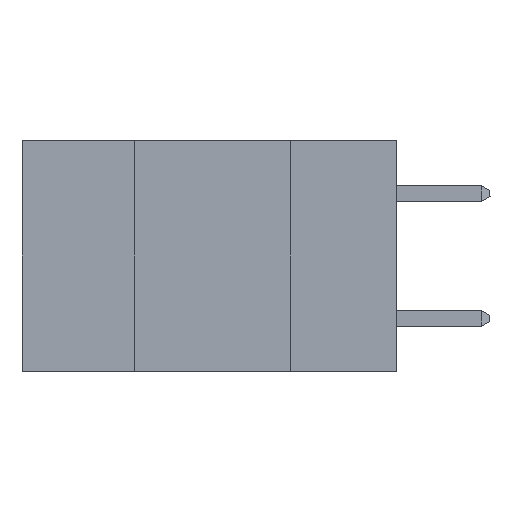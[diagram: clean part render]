
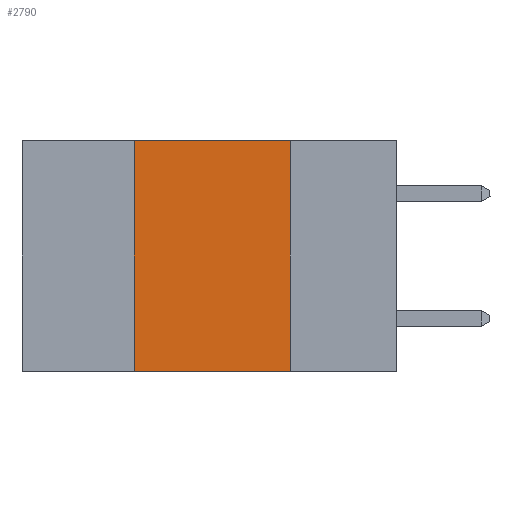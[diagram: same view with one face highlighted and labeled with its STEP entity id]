
A CAD part, left-side view. The second image highlights one B-rep face of the part: STEP entity #2790.
In plain terms, the highlighted planar face has unit normal (-1, 0, 0).
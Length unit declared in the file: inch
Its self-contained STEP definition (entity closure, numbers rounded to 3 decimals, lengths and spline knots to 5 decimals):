
#112 = CARTESIAN_POINT ( 'NONE',  ( 0., 0.42, 0. ) ) ;
#706 = ORIENTED_EDGE ( 'NONE', *, *, #27889, .F. ) ;
#2756 = CARTESIAN_POINT ( 'NONE',  ( 0., 0.6, 0. ) ) ;
#2790 = ADVANCED_FACE ( 'NONE', ( #22923 ), #14587, .F. ) ;
#3957 = CARTESIAN_POINT ( 'NONE',  ( 0., 0.17, -0.37 ) ) ;
#4171 = CARTESIAN_POINT ( 'NONE',  ( 0., 0.6, -0.37 ) ) ;
#4883 = LINE ( 'NONE', #4171, #29464 ) ;
#5131 = DIRECTION ( 'NONE',  ( 0., 0., -1. ) ) ;
#6451 = DIRECTION ( 'NONE',  ( 0., -1., 0. ) ) ;
#7254 = ORIENTED_EDGE ( 'NONE', *, *, #17502, .F. ) ;
#7613 = CARTESIAN_POINT ( 'NONE',  ( 0., 0.42, 0. ) ) ;
#9330 = ORIENTED_EDGE ( 'NONE', *, *, #13135, .T. ) ;
#9490 = CARTESIAN_POINT ( 'NONE',  ( 0., 0.6, 0. ) ) ;
#10013 = DIRECTION ( 'NONE',  ( 1., 0., 0. ) ) ;
#10082 = VERTEX_POINT ( 'NONE', #21929 ) ;
#13135 = EDGE_CURVE ( 'NONE', #26389, #22749, #4883, .T. ) ;
#14587 = PLANE ( 'NONE',  #16981 ) ;
#14871 = CARTESIAN_POINT ( 'NONE',  ( 0., 0.17, 0. ) ) ;
#16442 = LINE ( 'NONE', #9490, #21316 ) ;
#16981 = AXIS2_PLACEMENT_3D ( 'NONE', #2756, #10013, #5131 ) ;
#17502 = EDGE_CURVE ( 'NONE', #10082, #22749, #25184, .T. ) ;
#17795 = EDGE_CURVE ( 'NONE', #26389, #28243, #30003, .T. ) ;
#21316 = VECTOR ( 'NONE', #28324, 39.37008 ) ;
#21929 = CARTESIAN_POINT ( 'NONE',  ( 0., 0.17, 0. ) ) ;
#21950 = EDGE_LOOP ( 'NONE', ( #7254, #706, #22397, #9330 ) ) ;
#21998 = DIRECTION ( 'NONE',  ( 0., 0., 1. ) ) ;
#22397 = ORIENTED_EDGE ( 'NONE', *, *, #17795, .F. ) ;
#22561 = CARTESIAN_POINT ( 'NONE',  ( 0., 0.42, -0.37 ) ) ;
#22749 = VERTEX_POINT ( 'NONE', #3957 ) ;
#22923 = FACE_OUTER_BOUND ( 'NONE', #21950, .T. ) ;
#23325 = VECTOR ( 'NONE', #21998, 39.37008 ) ;
#25184 = LINE ( 'NONE', #14871, #30400 ) ;
#26389 = VERTEX_POINT ( 'NONE', #22561 ) ;
#26755 = DIRECTION ( 'NONE',  ( 0., 0., -1. ) ) ;
#27889 = EDGE_CURVE ( 'NONE', #28243, #10082, #16442, .T. ) ;
#28243 = VERTEX_POINT ( 'NONE', #112 ) ;
#28324 = DIRECTION ( 'NONE',  ( 0., -1., 0. ) ) ;
#29464 = VECTOR ( 'NONE', #6451, 39.37008 ) ;
#30003 = LINE ( 'NONE', #7613, #23325 ) ;
#30400 = VECTOR ( 'NONE', #26755, 39.37008 ) ;
